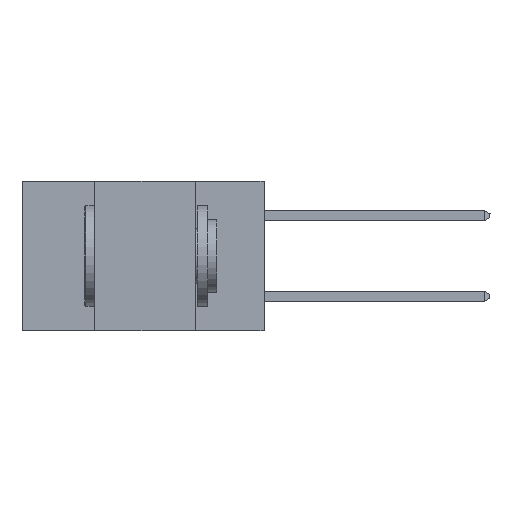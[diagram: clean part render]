
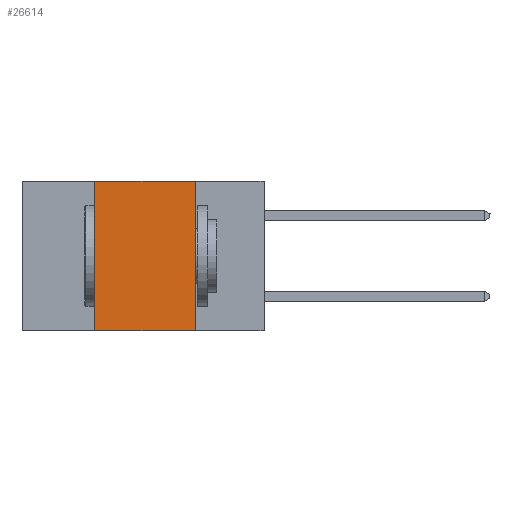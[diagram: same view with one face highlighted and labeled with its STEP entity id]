
A CAD part, left-side view. The second image highlights one B-rep face of the part: STEP entity #26614.
In plain terms, the highlighted planar face has unit normal (-1, 0, 0).
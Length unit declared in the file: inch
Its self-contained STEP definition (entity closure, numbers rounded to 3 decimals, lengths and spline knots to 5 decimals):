
#244 = ORIENTED_EDGE ( 'NONE', *, *, #21279, .F. ) ;
#2017 = EDGE_CURVE ( 'NONE', #6466, #2828, #12630, .T. ) ;
#2828 = VERTEX_POINT ( 'NONE', #7375 ) ;
#3383 = VECTOR ( 'NONE', #15898, 39.37008 ) ;
#3613 = CARTESIAN_POINT ( 'NONE',  ( 0., 0.17, -0.37 ) ) ;
#3973 = CARTESIAN_POINT ( 'NONE',  ( 0., 0.42, 0. ) ) ;
#4073 = VECTOR ( 'NONE', #27327, 39.37008 ) ;
#5971 = CARTESIAN_POINT ( 'NONE',  ( 0., 0.42, 0. ) ) ;
#6466 = VERTEX_POINT ( 'NONE', #5971 ) ;
#7375 = CARTESIAN_POINT ( 'NONE',  ( 0., 0.17, 0. ) ) ;
#8129 = CARTESIAN_POINT ( 'NONE',  ( 0., 0.6, 0. ) ) ;
#9000 = VECTOR ( 'NONE', #16121, 39.37008 ) ;
#10591 = AXIS2_PLACEMENT_3D ( 'NONE', #14994, #26473, #17352 ) ;
#11413 = EDGE_LOOP ( 'NONE', ( #244, #12887, #17426, #29644 ) ) ;
#11947 = LINE ( 'NONE', #3973, #3383 ) ;
#12630 = LINE ( 'NONE', #8129, #4073 ) ;
#12887 = ORIENTED_EDGE ( 'NONE', *, *, #2017, .F. ) ;
#14040 = CARTESIAN_POINT ( 'NONE',  ( 0., 0.6, -0.37 ) ) ;
#14994 = CARTESIAN_POINT ( 'NONE',  ( 0., 0.6, 0. ) ) ;
#15747 = DIRECTION ( 'NONE',  ( 0., 0., -1. ) ) ;
#15898 = DIRECTION ( 'NONE',  ( 0., 0., 1. ) ) ;
#15963 = VERTEX_POINT ( 'NONE', #3613 ) ;
#16121 = DIRECTION ( 'NONE',  ( 0., -1., 0. ) ) ;
#17134 = CARTESIAN_POINT ( 'NONE',  ( 0., 0.17, 0. ) ) ;
#17352 = DIRECTION ( 'NONE',  ( 0., 0., -1. ) ) ;
#17426 = ORIENTED_EDGE ( 'NONE', *, *, #19861, .F. ) ;
#18120 = CARTESIAN_POINT ( 'NONE',  ( 0., 0.42, -0.37 ) ) ;
#18669 = EDGE_CURVE ( 'NONE', #23719, #15963, #23878, .T. ) ;
#19861 = EDGE_CURVE ( 'NONE', #23719, #6466, #11947, .T. ) ;
#21279 = EDGE_CURVE ( 'NONE', #2828, #15963, #22647, .T. ) ;
#21512 = VECTOR ( 'NONE', #15747, 39.37008 ) ;
#22647 = LINE ( 'NONE', #17134, #21512 ) ;
#23719 = VERTEX_POINT ( 'NONE', #18120 ) ;
#23878 = LINE ( 'NONE', #14040, #9000 ) ;
#26256 = FACE_OUTER_BOUND ( 'NONE', #11413, .T. ) ;
#26473 = DIRECTION ( 'NONE',  ( 1., 0., 0. ) ) ;
#26614 = ADVANCED_FACE ( 'NONE', ( #26256 ), #28959, .F. ) ;
#27327 = DIRECTION ( 'NONE',  ( 0., -1., 0. ) ) ;
#28959 = PLANE ( 'NONE',  #10591 ) ;
#29644 = ORIENTED_EDGE ( 'NONE', *, *, #18669, .T. ) ;
